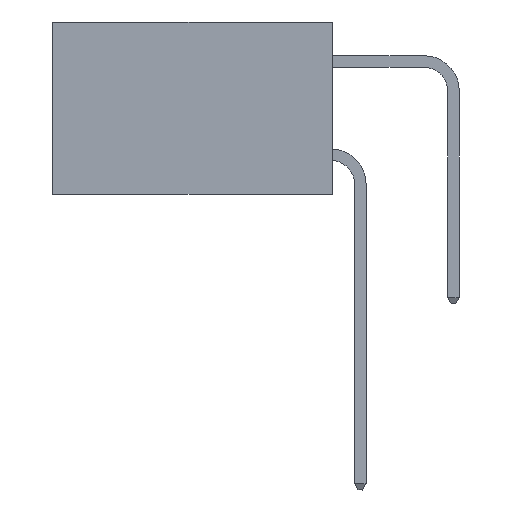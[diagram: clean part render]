
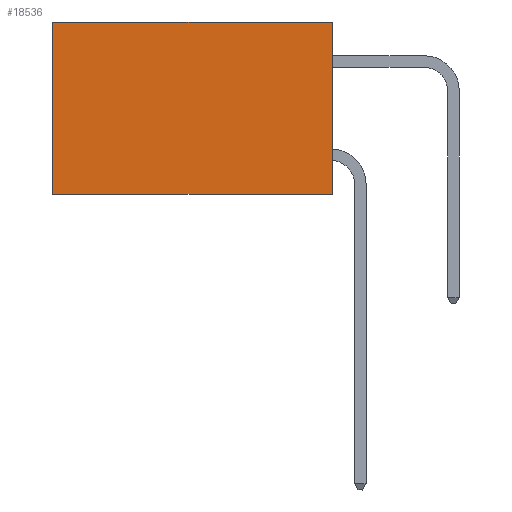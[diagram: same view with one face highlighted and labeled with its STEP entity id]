
A CAD part, left-side view. The second image highlights one B-rep face of the part: STEP entity #18536.
In plain terms, the highlighted planar face has unit normal (-1, 0, 0).
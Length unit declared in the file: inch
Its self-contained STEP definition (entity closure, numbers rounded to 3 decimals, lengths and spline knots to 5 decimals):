
#412 = CARTESIAN_POINT ( 'NONE',  ( 0.298, 0., 0. ) ) ;
#2365 = CARTESIAN_POINT ( 'NONE',  ( 0.298, 0., 0. ) ) ;
#2409 = VERTEX_POINT ( 'NONE', #3512 ) ;
#2429 = VERTEX_POINT ( 'NONE', #12381 ) ;
#2606 = DIRECTION ( 'NONE',  ( 1., 0., 0. ) ) ;
#2616 = VERTEX_POINT ( 'NONE', #8792 ) ;
#3512 = CARTESIAN_POINT ( 'NONE',  ( 0.298, 0., -0.37 ) ) ;
#3819 = DIRECTION ( 'NONE',  ( 0., 0., -1. ) ) ;
#3971 = EDGE_CURVE ( 'NONE', #2409, #2616, #18316, .T. ) ;
#4981 = VECTOR ( 'NONE', #18693, 39.37008 ) ;
#5444 = VECTOR ( 'NONE', #9299, 39.37008 ) ;
#5905 = ORIENTED_EDGE ( 'NONE', *, *, #12312, .F. ) ;
#5974 = CARTESIAN_POINT ( 'NONE',  ( 0.298, 0., 0. ) ) ;
#7024 = VECTOR ( 'NONE', #3819, 39.37008 ) ;
#8019 = ORIENTED_EDGE ( 'NONE', *, *, #15274, .T. ) ;
#8104 = EDGE_LOOP ( 'NONE', ( #19844, #12689, #5905, #8019 ) ) ;
#8792 = CARTESIAN_POINT ( 'NONE',  ( 0.298, 0.6, -0.37 ) ) ;
#9299 = DIRECTION ( 'NONE',  ( 0., 1., 0. ) ) ;
#9478 = LINE ( 'NONE', #2365, #4981 ) ;
#10514 = CARTESIAN_POINT ( 'NONE',  ( 0.298, 0., -0.37 ) ) ;
#10590 = CARTESIAN_POINT ( 'NONE',  ( 0.298, 0., 0. ) ) ;
#10886 = LINE ( 'NONE', #10590, #7024 ) ;
#11032 = VERTEX_POINT ( 'NONE', #412 ) ;
#11120 = AXIS2_PLACEMENT_3D ( 'NONE', #5974, #2606, #14227 ) ;
#11712 = VECTOR ( 'NONE', #18007, 39.37008 ) ;
#12312 = EDGE_CURVE ( 'NONE', #11032, #2409, #10886, .T. ) ;
#12381 = CARTESIAN_POINT ( 'NONE',  ( 0.298, 0.6, 0. ) ) ;
#12596 = PLANE ( 'NONE',  #11120 ) ;
#12689 = ORIENTED_EDGE ( 'NONE', *, *, #3971, .F. ) ;
#14227 = DIRECTION ( 'NONE',  ( 0., 0., -1. ) ) ;
#15274 = EDGE_CURVE ( 'NONE', #11032, #2429, #9478, .T. ) ;
#15964 = LINE ( 'NONE', #16474, #11712 ) ;
#16474 = CARTESIAN_POINT ( 'NONE',  ( 0.298, 0.6, 0. ) ) ;
#16936 = EDGE_CURVE ( 'NONE', #2429, #2616, #15964, .T. ) ;
#18007 = DIRECTION ( 'NONE',  ( 0., 0., -1. ) ) ;
#18316 = LINE ( 'NONE', #10514, #5444 ) ;
#18536 = ADVANCED_FACE ( 'NONE', ( #20556 ), #12596, .F. ) ;
#18693 = DIRECTION ( 'NONE',  ( 0., 1., 0. ) ) ;
#19844 = ORIENTED_EDGE ( 'NONE', *, *, #16936, .T. ) ;
#20556 = FACE_OUTER_BOUND ( 'NONE', #8104, .T. ) ;
